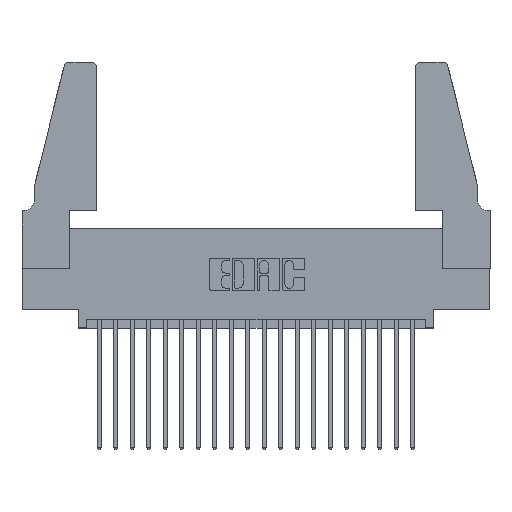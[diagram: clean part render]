
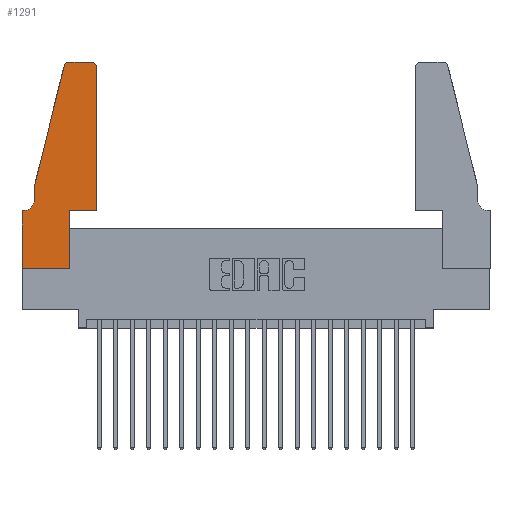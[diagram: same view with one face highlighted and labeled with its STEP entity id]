
A CAD part, top view. The second image highlights one B-rep face of the part: STEP entity #1291.
In plain terms, the highlighted planar face has unit normal (0, 0, 1).
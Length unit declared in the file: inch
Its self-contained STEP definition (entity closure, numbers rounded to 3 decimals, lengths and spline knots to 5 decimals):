
#863 = EDGE_CURVE ( 'NONE', #4430, #1610, #13961, .T. ) ;
#930 = CARTESIAN_POINT ( 'NONE',  ( 0., 0.35, 0.37 ) ) ;
#979 = LINE ( 'NONE', #11633, #14654 ) ;
#1291 = ADVANCED_FACE ( 'NONE', ( #1752 ), #15752, .T. ) ;
#1513 = VECTOR ( 'NONE', #19249, 39.37008 ) ;
#1610 = VERTEX_POINT ( 'NONE', #10697 ) ;
#1748 = DIRECTION ( 'NONE',  ( 0., -1., 0. ) ) ;
#1752 = FACE_OUTER_BOUND ( 'NONE', #4814, .T. ) ;
#1998 = LINE ( 'NONE', #16743, #1513 ) ;
#2071 = EDGE_CURVE ( 'NONE', #8122, #4430, #19629, .T. ) ;
#2623 = CARTESIAN_POINT ( 'NONE',  ( 0.2865, 0., 0.37 ) ) ;
#2668 = AXIS2_PLACEMENT_3D ( 'NONE', #12940, #8265, #3239 ) ;
#2721 = CARTESIAN_POINT ( 'NONE',  ( 0.284, 1.25, 0.37 ) ) ;
#3004 = EDGE_CURVE ( 'NONE', #9410, #11480, #20870, .T. ) ;
#3201 = ORIENTED_EDGE ( 'NONE', *, *, #2071, .T. ) ;
#3239 = DIRECTION ( 'NONE',  ( 1., 0., 0. ) ) ;
#3271 = ORIENTED_EDGE ( 'NONE', *, *, #4427, .T. ) ;
#3309 = AXIS2_PLACEMENT_3D ( 'NONE', #18514, #18369, #12012 ) ;
#3598 = VECTOR ( 'NONE', #11955, 39.37008 ) ;
#3644 = VERTEX_POINT ( 'NONE', #930 ) ;
#3746 = VECTOR ( 'NONE', #14928, 39.37008 ) ;
#4117 = ORIENTED_EDGE ( 'NONE', *, *, #3004, .T. ) ;
#4276 = VERTEX_POINT ( 'NONE', #14516 ) ;
#4427 = EDGE_CURVE ( 'NONE', #8926, #3644, #1998, .T. ) ;
#4430 = VERTEX_POINT ( 'NONE', #12004 ) ;
#4814 = EDGE_LOOP ( 'NONE', ( #4117, #6731, #18284, #12112, #5744, #3271, #5019, #18986, #15582, #3201, #16544, #13278 ) ) ;
#4988 = EDGE_CURVE ( 'NONE', #6713, #6289, #979, .T. ) ;
#5019 = ORIENTED_EDGE ( 'NONE', *, *, #8266, .T. ) ;
#5328 = EDGE_CURVE ( 'NONE', #4276, #6445, #11122, .T. ) ;
#5744 = ORIENTED_EDGE ( 'NONE', *, *, #7857, .T. ) ;
#5978 = CARTESIAN_POINT ( 'NONE',  ( 0.0755, 0.5, 0.37 ) ) ;
#6057 = DIRECTION ( 'NONE',  ( 1., 0., 0. ) ) ;
#6209 = VECTOR ( 'NONE', #6057, 39.37008 ) ;
#6289 = VERTEX_POINT ( 'NONE', #13378 ) ;
#6347 = CARTESIAN_POINT ( 'NONE',  ( 0.4205, 1.25, 0.37 ) ) ;
#6445 = VERTEX_POINT ( 'NONE', #2623 ) ;
#6450 = VECTOR ( 'NONE', #1748, 39.37008 ) ;
#6635 = DIRECTION ( 'NONE',  ( -1., 0., 0. ) ) ;
#6713 = VERTEX_POINT ( 'NONE', #5978 ) ;
#6731 = ORIENTED_EDGE ( 'NONE', *, *, #8629, .T. ) ;
#6874 = CIRCLE ( 'NONE', #12240, 0.07 ) ;
#7234 = EDGE_CURVE ( 'NONE', #7445, #6713, #8026, .T. ) ;
#7445 = VERTEX_POINT ( 'NONE', #20009 ) ;
#7857 = EDGE_CURVE ( 'NONE', #6289, #8926, #6874, .T. ) ;
#8026 = LINE ( 'NONE', #18888, #14348 ) ;
#8122 = VERTEX_POINT ( 'NONE', #10477 ) ;
#8265 = DIRECTION ( 'NONE',  ( 0., 0., 1. ) ) ;
#8266 = EDGE_CURVE ( 'NONE', #3644, #4276, #10248, .T. ) ;
#8384 = CARTESIAN_POINT ( 'NONE',  ( 0., 0., 0.37 ) ) ;
#8629 = EDGE_CURVE ( 'NONE', #11480, #7445, #13763, .T. ) ;
#8926 = VERTEX_POINT ( 'NONE', #10979 ) ;
#9410 = VERTEX_POINT ( 'NONE', #6347 ) ;
#10248 = LINE ( 'NONE', #19911, #6450 ) ;
#10477 = CARTESIAN_POINT ( 'NONE',  ( 0.2865, 0.35, 0.37 ) ) ;
#10697 = CARTESIAN_POINT ( 'NONE',  ( 0.4505, 1.22, 0.37 ) ) ;
#10791 = CARTESIAN_POINT ( 'NONE',  ( 0.2865, 0.35, 0.37 ) ) ;
#10979 = CARTESIAN_POINT ( 'NONE',  ( 0.0055, 0.35, 0.37 ) ) ;
#11122 = LINE ( 'NONE', #8384, #3746 ) ;
#11352 = LINE ( 'NONE', #10791, #12376 ) ;
#11480 = VERTEX_POINT ( 'NONE', #2721 ) ;
#11541 = CIRCLE ( 'NONE', #2668, 0.03 ) ;
#11633 = CARTESIAN_POINT ( 'NONE',  ( 0.0755, 0.5, 0.37 ) ) ;
#11955 = DIRECTION ( 'NONE',  ( -1., 0., 0. ) ) ;
#12004 = CARTESIAN_POINT ( 'NONE',  ( 0.4505, 0.35, 0.37 ) ) ;
#12012 = DIRECTION ( 'NONE',  ( 1., 0., 0. ) ) ;
#12112 = ORIENTED_EDGE ( 'NONE', *, *, #4988, .T. ) ;
#12240 = AXIS2_PLACEMENT_3D ( 'NONE', #20071, #20904, #6635 ) ;
#12342 = DIRECTION ( 'NONE',  ( 1., 0., 0. ) ) ;
#12376 = VECTOR ( 'NONE', #17334, 39.37008 ) ;
#12940 = CARTESIAN_POINT ( 'NONE',  ( 0.4205, 1.22, 0.37 ) ) ;
#13278 = ORIENTED_EDGE ( 'NONE', *, *, #14089, .T. ) ;
#13351 = AXIS2_PLACEMENT_3D ( 'NONE', #20925, #20140, #12342 ) ;
#13378 = CARTESIAN_POINT ( 'NONE',  ( 0.0755, 0.42, 0.37 ) ) ;
#13496 = CARTESIAN_POINT ( 'NONE',  ( 0.2605, 1.25, 0.37 ) ) ;
#13763 = CIRCLE ( 'NONE', #3309, 0.03 ) ;
#13961 = LINE ( 'NONE', #19741, #15983 ) ;
#14089 = EDGE_CURVE ( 'NONE', #1610, #9410, #11541, .T. ) ;
#14348 = VECTOR ( 'NONE', #20679, 39.37008 ) ;
#14516 = CARTESIAN_POINT ( 'NONE',  ( 0., 0., 0.37 ) ) ;
#14654 = VECTOR ( 'NONE', #14674, 39.37008 ) ;
#14674 = DIRECTION ( 'NONE',  ( 0., -1., 0. ) ) ;
#14928 = DIRECTION ( 'NONE',  ( 1., 0., 0. ) ) ;
#15582 = ORIENTED_EDGE ( 'NONE', *, *, #15885, .T. ) ;
#15752 = PLANE ( 'NONE',  #13351 ) ;
#15885 = EDGE_CURVE ( 'NONE', #6445, #8122, #11352, .T. ) ;
#15983 = VECTOR ( 'NONE', #20220, 39.37008 ) ;
#16544 = ORIENTED_EDGE ( 'NONE', *, *, #863, .T. ) ;
#16743 = CARTESIAN_POINT ( 'NONE',  ( 0.0755, 0.35, 0.37 ) ) ;
#17334 = DIRECTION ( 'NONE',  ( 0., 1., 0. ) ) ;
#18284 = ORIENTED_EDGE ( 'NONE', *, *, #7234, .T. ) ;
#18369 = DIRECTION ( 'NONE',  ( 0., 0., 1. ) ) ;
#18514 = CARTESIAN_POINT ( 'NONE',  ( 0.284, 1.22, 0.37 ) ) ;
#18888 = CARTESIAN_POINT ( 'NONE',  ( 0.0755, 0.5, 0.37 ) ) ;
#18986 = ORIENTED_EDGE ( 'NONE', *, *, #5328, .T. ) ;
#19249 = DIRECTION ( 'NONE',  ( -1., 0., 0. ) ) ;
#19295 = CARTESIAN_POINT ( 'NONE',  ( 0.4505, 0.35, 0.37 ) ) ;
#19629 = LINE ( 'NONE', #19295, #6209 ) ;
#19741 = CARTESIAN_POINT ( 'NONE',  ( 0.4505, 0.35, 0.37 ) ) ;
#19911 = CARTESIAN_POINT ( 'NONE',  ( 0., 0., 0.37 ) ) ;
#20009 = CARTESIAN_POINT ( 'NONE',  ( 0.25487, 1.22718, 0.37 ) ) ;
#20071 = CARTESIAN_POINT ( 'NONE',  ( 0.0055, 0.42, 0.37 ) ) ;
#20140 = DIRECTION ( 'NONE',  ( 0., 0., 1. ) ) ;
#20220 = DIRECTION ( 'NONE',  ( 0., 1., 0. ) ) ;
#20679 = DIRECTION ( 'NONE',  ( -0.239, -0.971, 0. ) ) ;
#20870 = LINE ( 'NONE', #13496, #3598 ) ;
#20904 = DIRECTION ( 'NONE',  ( 0., 0., -1. ) ) ;
#20925 = CARTESIAN_POINT ( 'NONE',  ( 0., 0.35, 0.37 ) ) ;
